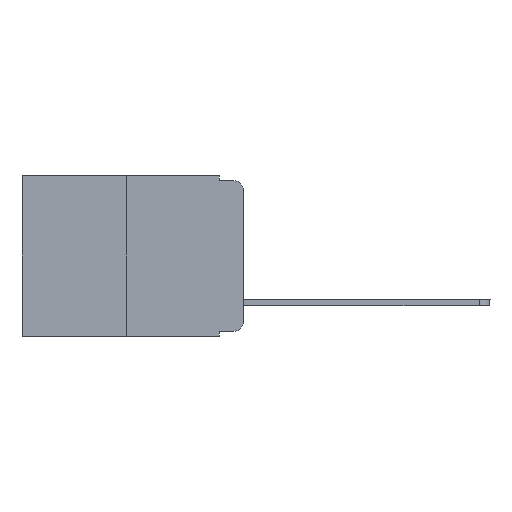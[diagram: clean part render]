
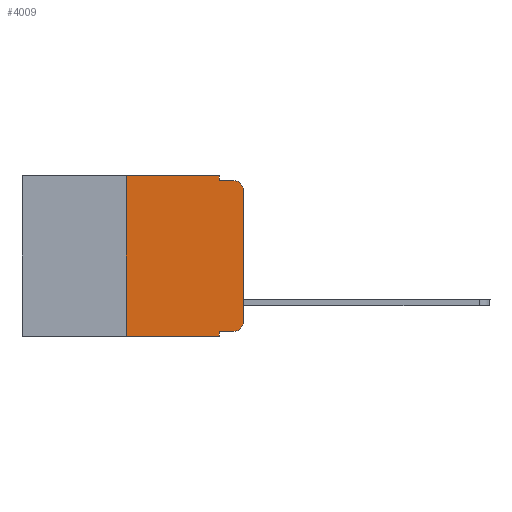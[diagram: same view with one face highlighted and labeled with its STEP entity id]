
A CAD part, left-side view. The second image highlights one B-rep face of the part: STEP entity #4009.
In plain terms, the highlighted planar face has unit normal (-1, 0, 0).
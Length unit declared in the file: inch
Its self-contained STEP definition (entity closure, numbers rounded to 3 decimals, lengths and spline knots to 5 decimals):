
#271 = CARTESIAN_POINT ( 'NONE',  ( 0., 0., -0.03 ) ) ;
#356 = DIRECTION ( 'NONE',  ( -1., 0., 0. ) ) ;
#2014 = VERTEX_POINT ( 'NONE', #4856 ) ;
#2054 = DIRECTION ( 'NONE',  ( 0., 0., -1. ) ) ;
#2536 = CARTESIAN_POINT ( 'NONE',  ( 0., 0.25, 0. ) ) ;
#2682 = DIRECTION ( 'NONE',  ( -1., 0., 0. ) ) ;
#2816 = ORIENTED_EDGE ( 'NONE', *, *, #5445, .F. ) ;
#3017 = DIRECTION ( 'NONE',  ( 0., 0., -1. ) ) ;
#3241 = CARTESIAN_POINT ( 'NONE',  ( 0., 0.051, 0. ) ) ;
#3308 = CARTESIAN_POINT ( 'NONE',  ( 0., 0.473, -0.343 ) ) ;
#3337 = VECTOR ( 'NONE', #6278, 39.37008 ) ;
#3349 = VERTEX_POINT ( 'NONE', #19923 ) ;
#3427 = EDGE_CURVE ( 'NONE', #15471, #3349, #13983, .T. ) ;
#3725 = LINE ( 'NONE', #3953, #12238 ) ;
#3814 = VECTOR ( 'NONE', #16542, 39.37008 ) ;
#3953 = CARTESIAN_POINT ( 'NONE',  ( 0., 0.051, -0.333 ) ) ;
#4009 = ADVANCED_FACE ( 'NONE', ( #21672 ), #16102, .F. ) ;
#4249 = LINE ( 'NONE', #2536, #3814 ) ;
#4332 = VERTEX_POINT ( 'NONE', #16285 ) ;
#4359 = DIRECTION ( 'NONE',  ( 0., 0., -1. ) ) ;
#4518 = CARTESIAN_POINT ( 'NONE',  ( 0., 0., 0. ) ) ;
#4587 = ORIENTED_EDGE ( 'NONE', *, *, #20377, .T. ) ;
#4622 = CARTESIAN_POINT ( 'NONE',  ( 0., 0.02, -0.03 ) ) ;
#4856 = CARTESIAN_POINT ( 'NONE',  ( 0., 0.02, -0.01 ) ) ;
#4928 = EDGE_CURVE ( 'NONE', #22011, #8117, #18290, .T. ) ;
#4983 = ORIENTED_EDGE ( 'NONE', *, *, #17894, .T. ) ;
#5435 = VECTOR ( 'NONE', #16976, 39.37008 ) ;
#5442 = CARTESIAN_POINT ( 'NONE',  ( 0., 0., -0.313 ) ) ;
#5445 = EDGE_CURVE ( 'NONE', #12970, #2014, #21980, .T. ) ;
#5496 = VERTEX_POINT ( 'NONE', #14113 ) ;
#5746 = CARTESIAN_POINT ( 'NONE',  ( 0., 0.25, 0. ) ) ;
#5963 = CARTESIAN_POINT ( 'NONE',  ( 0., 0.473, 0. ) ) ;
#6028 = LINE ( 'NONE', #13084, #8986 ) ;
#6069 = DIRECTION ( 'NONE',  ( 1., 0., 0. ) ) ;
#6278 = DIRECTION ( 'NONE',  ( 0., -1., 0. ) ) ;
#8117 = VERTEX_POINT ( 'NONE', #271 ) ;
#8176 = VERTEX_POINT ( 'NONE', #5746 ) ;
#8491 = DIRECTION ( 'NONE',  ( 0., 0., -1. ) ) ;
#8986 = VECTOR ( 'NONE', #11264, 39.37008 ) ;
#9272 = CIRCLE ( 'NONE', #12165, 0.02 ) ;
#9444 = EDGE_CURVE ( 'NONE', #17722, #8176, #4249, .T. ) ;
#9446 = AXIS2_PLACEMENT_3D ( 'NONE', #14116, #356, #2054 ) ;
#9506 = CARTESIAN_POINT ( 'NONE',  ( 0., 0.051, -0.01 ) ) ;
#10166 = ORIENTED_EDGE ( 'NONE', *, *, #12780, .F. ) ;
#10912 = DIRECTION ( 'NONE',  ( 0., -1., 0. ) ) ;
#11264 = DIRECTION ( 'NONE',  ( 0., -1., 0. ) ) ;
#11637 = ORIENTED_EDGE ( 'NONE', *, *, #13921, .T. ) ;
#11769 = ORIENTED_EDGE ( 'NONE', *, *, #20268, .T. ) ;
#12165 = AXIS2_PLACEMENT_3D ( 'NONE', #4622, #2682, #3017 ) ;
#12167 = DIRECTION ( 'NONE',  ( 0., 0., -1. ) ) ;
#12238 = VECTOR ( 'NONE', #10912, 39.37008 ) ;
#12780 = EDGE_CURVE ( 'NONE', #5496, #12970, #18844, .T. ) ;
#12970 = VERTEX_POINT ( 'NONE', #9506 ) ;
#13084 = CARTESIAN_POINT ( 'NONE',  ( 0., 0.473, 0. ) ) ;
#13148 = VECTOR ( 'NONE', #20337, 39.37008 ) ;
#13340 = CARTESIAN_POINT ( 'NONE',  ( 0., 0.051, -0.01 ) ) ;
#13421 = ORIENTED_EDGE ( 'NONE', *, *, #4928, .T. ) ;
#13921 = EDGE_CURVE ( 'NONE', #8117, #2014, #9272, .T. ) ;
#13983 = LINE ( 'NONE', #22293, #18550 ) ;
#14113 = CARTESIAN_POINT ( 'NONE',  ( 0., 0.051, 0. ) ) ;
#14116 = CARTESIAN_POINT ( 'NONE',  ( 0., 0.02, -0.313 ) ) ;
#15471 = VERTEX_POINT ( 'NONE', #18056 ) ;
#16079 = ORIENTED_EDGE ( 'NONE', *, *, #17537, .F. ) ;
#16102 = PLANE ( 'NONE',  #21834 ) ;
#16285 = CARTESIAN_POINT ( 'NONE',  ( 0., 0.02, -0.333 ) ) ;
#16542 = DIRECTION ( 'NONE',  ( 0., 0., 1. ) ) ;
#16865 = LINE ( 'NONE', #3308, #5435 ) ;
#16976 = DIRECTION ( 'NONE',  ( 0., -1., 0. ) ) ;
#17168 = CARTESIAN_POINT ( 'NONE',  ( 0., 0.25, -0.343 ) ) ;
#17537 = EDGE_CURVE ( 'NONE', #8176, #5496, #6028, .T. ) ;
#17722 = VERTEX_POINT ( 'NONE', #17168 ) ;
#17894 = EDGE_CURVE ( 'NONE', #15471, #4332, #3725, .T. ) ;
#18056 = CARTESIAN_POINT ( 'NONE',  ( 0., 0.051, -0.333 ) ) ;
#18290 = LINE ( 'NONE', #4518, #13148 ) ;
#18550 = VECTOR ( 'NONE', #12167, 39.37008 ) ;
#18844 = LINE ( 'NONE', #3241, #19623 ) ;
#19097 = ORIENTED_EDGE ( 'NONE', *, *, #3427, .F. ) ;
#19623 = VECTOR ( 'NONE', #8491, 39.37008 ) ;
#19633 = EDGE_LOOP ( 'NONE', ( #13421, #11637, #2816, #10166, #16079, #21540, #11769, #19097, #4983, #4587 ) ) ;
#19923 = CARTESIAN_POINT ( 'NONE',  ( 0., 0.051, -0.343 ) ) ;
#20268 = EDGE_CURVE ( 'NONE', #17722, #3349, #16865, .T. ) ;
#20337 = DIRECTION ( 'NONE',  ( 0., 0., 1. ) ) ;
#20377 = EDGE_CURVE ( 'NONE', #4332, #22011, #20711, .T. ) ;
#20711 = CIRCLE ( 'NONE', #9446, 0.02 ) ;
#21540 = ORIENTED_EDGE ( 'NONE', *, *, #9444, .F. ) ;
#21672 = FACE_OUTER_BOUND ( 'NONE', #19633, .T. ) ;
#21834 = AXIS2_PLACEMENT_3D ( 'NONE', #5963, #6069, #4359 ) ;
#21980 = LINE ( 'NONE', #13340, #3337 ) ;
#22011 = VERTEX_POINT ( 'NONE', #5442 ) ;
#22293 = CARTESIAN_POINT ( 'NONE',  ( 0., 0.051, 0. ) ) ;
